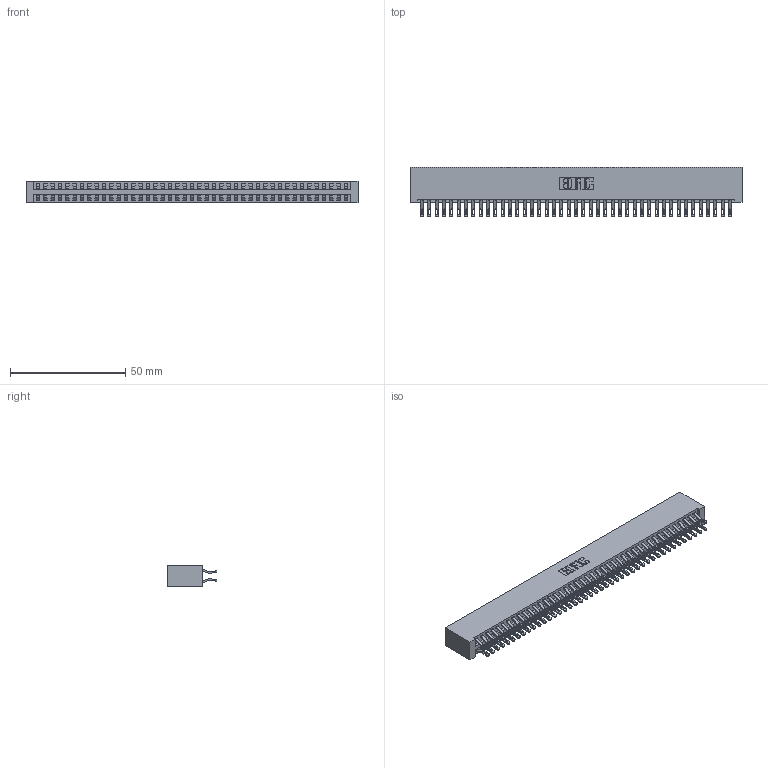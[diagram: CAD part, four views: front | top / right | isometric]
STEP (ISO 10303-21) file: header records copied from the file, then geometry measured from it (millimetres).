
FILE_DESCRIPTION (( 'STEP AP203' ), '1' );
FILE_NAME ('346-086-555-201.STEP', '2018-08-29T22:55:31', ( '' ), ( '' ), 'SwSTEP 2.0', 'SolidWorks 2016', '' );
FILE_SCHEMA (( 'CONFIG_CONTROL_DESIGN' ));
Length unit declared in the file: inch
Products named in the file (3): 346 Part_No Mounting Lugs; 345-292-001_555 Tail; 346-086-555-201
Assembly tree (87 placements, depth 2):
  346-086-555-201
    346 Part_No Mounting Lugs
    345-292-001_555 Tail  x86
Bounding box: 143.76 x 21.46 x 9.4 mm (x, y, z)
Volume: 14849.3 mm3; surface area: 21479.4 mm2
Topology: 87 solids, 87 shells, 5102 faces, 16043 edges, 10694 vertices
Faces by surface type: plane 2910, cylinder 2192
Entity records: 27977 total; most frequent: CARTESIAN_POINT 4642, ORIENTED_EDGE 4546, DIRECTION 4105, EDGE_CURVE 2273, VECTOR 1957, LINE 1957, VERTEX_POINT 1514, AXIS2_PLACEMENT_3D 1074
